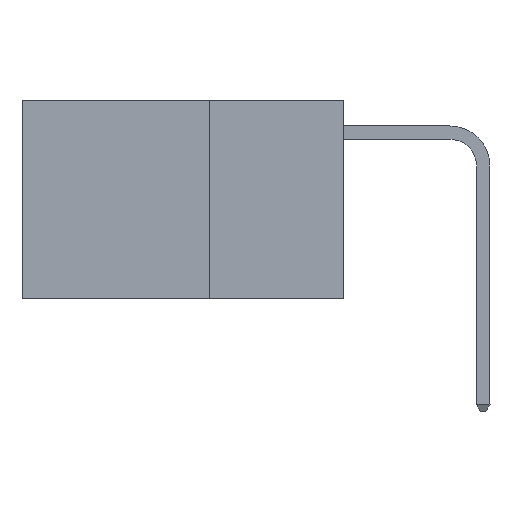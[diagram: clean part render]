
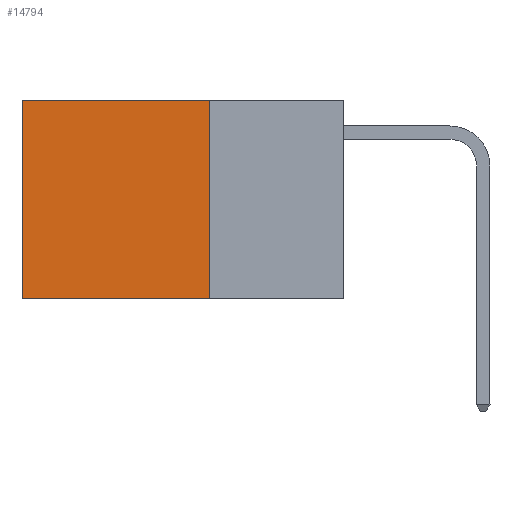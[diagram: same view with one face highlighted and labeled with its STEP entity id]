
A CAD part, left-side view. The second image highlights one B-rep face of the part: STEP entity #14794.
In plain terms, the highlighted planar face has unit normal (-1, 0, 0).
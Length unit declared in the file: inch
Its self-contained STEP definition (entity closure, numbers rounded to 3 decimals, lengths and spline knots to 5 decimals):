
#358 = EDGE_CURVE ( 'NONE', #6224, #3836, #12924, .T. ) ;
#600 = ORIENTED_EDGE ( 'NONE', *, *, #1286, .F. ) ;
#1050 = CARTESIAN_POINT ( 'NONE',  ( 0.2625, 0.25, -0.37 ) ) ;
#1286 = EDGE_CURVE ( 'NONE', #11104, #3836, #3975, .T. ) ;
#1948 = CARTESIAN_POINT ( 'NONE',  ( 0.2625, 0.6, 0. ) ) ;
#2791 = VECTOR ( 'NONE', #12822, 39.37008 ) ;
#3836 = VERTEX_POINT ( 'NONE', #9658 ) ;
#3975 = LINE ( 'NONE', #19853, #2791 ) ;
#6224 = VERTEX_POINT ( 'NONE', #1948 ) ;
#6372 = DIRECTION ( 'NONE',  ( 0., 0., -1. ) ) ;
#6484 = ORIENTED_EDGE ( 'NONE', *, *, #16614, .F. ) ;
#8076 = VECTOR ( 'NONE', #6372, 39.37008 ) ;
#8233 = PLANE ( 'NONE',  #12835 ) ;
#9613 = DIRECTION ( 'NONE',  ( 0., 1., 0. ) ) ;
#9658 = CARTESIAN_POINT ( 'NONE',  ( 0.2625, 0.6, -0.37 ) ) ;
#9686 = DIRECTION ( 'NONE',  ( 0., 0., -1. ) ) ;
#9985 = CARTESIAN_POINT ( 'NONE',  ( 0.2625, 0.6, 0. ) ) ;
#10070 = DIRECTION ( 'NONE',  ( 1., 0., 0. ) ) ;
#10815 = LINE ( 'NONE', #20349, #18043 ) ;
#11104 = VERTEX_POINT ( 'NONE', #1050 ) ;
#11131 = LINE ( 'NONE', #18510, #20007 ) ;
#11741 = EDGE_LOOP ( 'NONE', ( #19134, #600, #6484, #14558 ) ) ;
#11751 = FACE_OUTER_BOUND ( 'NONE', #11741, .T. ) ;
#12822 = DIRECTION ( 'NONE',  ( 0., 1., 0. ) ) ;
#12835 = AXIS2_PLACEMENT_3D ( 'NONE', #17181, #10070, #22475 ) ;
#12924 = LINE ( 'NONE', #9985, #8076 ) ;
#14558 = ORIENTED_EDGE ( 'NONE', *, *, #22212, .T. ) ;
#14794 = ADVANCED_FACE ( 'NONE', ( #11751 ), #8233, .F. ) ;
#16614 = EDGE_CURVE ( 'NONE', #21245, #11104, #10815, .T. ) ;
#17181 = CARTESIAN_POINT ( 'NONE',  ( 0.2625, 0.25, 0. ) ) ;
#17678 = CARTESIAN_POINT ( 'NONE',  ( 0.2625, 0.25, 0. ) ) ;
#18043 = VECTOR ( 'NONE', #9686, 39.37008 ) ;
#18510 = CARTESIAN_POINT ( 'NONE',  ( 0.2625, 0.25, 0. ) ) ;
#19134 = ORIENTED_EDGE ( 'NONE', *, *, #358, .T. ) ;
#19853 = CARTESIAN_POINT ( 'NONE',  ( 0.2625, 0.25, -0.37 ) ) ;
#20007 = VECTOR ( 'NONE', #9613, 39.37008 ) ;
#20349 = CARTESIAN_POINT ( 'NONE',  ( 0.2625, 0.25, 0. ) ) ;
#21245 = VERTEX_POINT ( 'NONE', #17678 ) ;
#22212 = EDGE_CURVE ( 'NONE', #21245, #6224, #11131, .T. ) ;
#22475 = DIRECTION ( 'NONE',  ( 0., 0., -1. ) ) ;
